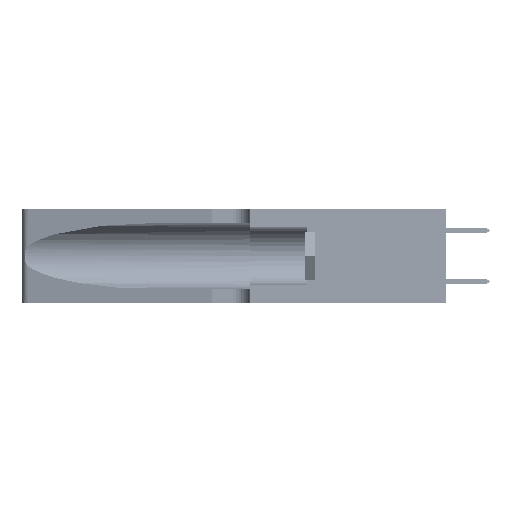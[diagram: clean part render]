
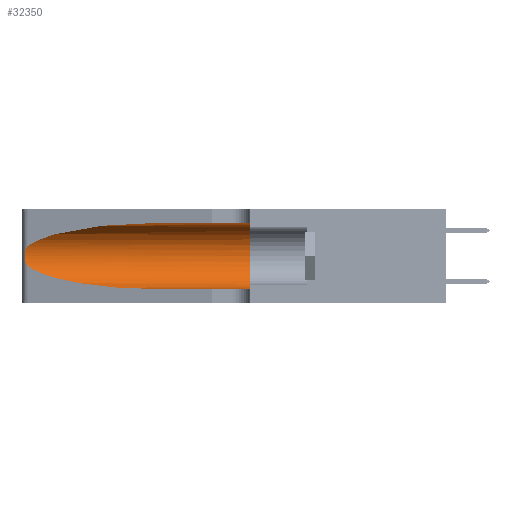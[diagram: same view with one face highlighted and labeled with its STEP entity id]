
A CAD part, left-side view. The second image highlights one B-rep face of the part: STEP entity #32350.
In plain terms, the highlighted cylindrical face has radius 3.308 mm (diameter 6.617 mm), a partial arc.
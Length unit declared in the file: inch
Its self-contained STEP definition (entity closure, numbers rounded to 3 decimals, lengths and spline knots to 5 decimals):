
#1364 = VERTEX_POINT ( 'NONE', #30475 ) ;
#2214 = CARTESIAN_POINT ( 'NONE',  ( 0.26075, 1.23896, 0.19203 ) ) ;
#2398 = CARTESIAN_POINT ( 'NONE',  ( 0.26017, 1.23833, 0.17102 ) ) ;
#4324 = FACE_OUTER_BOUND ( 'NONE', #38369, .T. ) ;
#5313 = CARTESIAN_POINT ( 'NONE',  ( 0.25487, 1.22718, 0.14631 ) ) ;
#6065 = EDGE_CURVE ( 'NONE', #1364, #43040, #25121, .T. ) ;
#6328 = CARTESIAN_POINT ( 'NONE',  ( 0.26075, 1.23896, 0.178 ) ) ;
#8182 = ORIENTED_EDGE ( 'NONE', *, *, #6065, .T. ) ;
#8504 = LINE ( 'NONE', #25974, #45544 ) ;
#8537 = AXIS2_PLACEMENT_3D ( 'NONE', #38284, #22401, #14534 ) ;
#9235 = CARTESIAN_POINT ( 'NONE',  ( 0.2373, 1.15595, 0.08982 ) ) ;
#9732 = CARTESIAN_POINT ( 'NONE',  ( 0.25639, 1.23186, 0.15144 ) ) ;
#9912 = CARTESIAN_POINT ( 'NONE',  ( 0.25789, 1.23486, 0.15765 ) ) ;
#14534 = DIRECTION ( 'NONE',  ( 0., 0., 1. ) ) ;
#15057 = ORIENTED_EDGE ( 'NONE', *, *, #47075, .T. ) ;
#15296 = CARTESIAN_POINT ( 'NONE',  ( 0.2373, 1.15595, 0.28018 ) ) ;
#15725 = CIRCLE ( 'NONE', #8537, 0.13025 ) ;
#16176 = CARTESIAN_POINT ( 'NONE',  ( 0.1305, 0.35, 0.05475 ) ) ;
#16829 = VERTEX_POINT ( 'NONE', #16176 ) ;
#17794 = DIRECTION ( 'NONE',  ( 0., -1., 0. ) ) ;
#18104 = CARTESIAN_POINT ( 'NONE',  ( 0.25555, 1.22994, 0.2215 ) ) ;
#18462 = CARTESIAN_POINT ( 'NONE',  ( 0.25487, 1.22718, 0.22369 ) ) ;
#18672 = EDGE_CURVE ( 'NONE', #46825, #24835, #45081, .T. ) ;
#20918 = CYLINDRICAL_SURFACE ( 'NONE', #23508, 0.13025 ) ;
#21162 = CARTESIAN_POINT ( 'NONE',  ( 0.1305, 1.61858, 0.05475 ) ) ;
#21567 = CARTESIAN_POINT ( 'NONE',  ( 0.18966, 0.96281, 0.05475 ) ) ;
#22038 = DIRECTION ( 'NONE',  ( 0., -1., 0. ) ) ;
#22401 = DIRECTION ( 'NONE',  ( 0., 1., 0. ) ) ;
#22582 = CARTESIAN_POINT ( 'NONE',  ( 0.25856, 1.23593, 0.16098 ) ) ;
#23114 = ORIENTED_EDGE ( 'NONE', *, *, #18672, .T. ) ;
#23508 = AXIS2_PLACEMENT_3D ( 'NONE', #42063, #17794, #31004 ) ;
#24835 = VERTEX_POINT ( 'NONE', #51493 ) ;
#24885 = ORIENTED_EDGE ( 'NONE', *, *, #35808, .F. ) ;
#25121 =( BOUNDED_CURVE ( )  B_SPLINE_CURVE ( 3, ( #5313, #9235, #21567, #42420 ),
 .UNSPECIFIED., .F., .F. ) 
 B_SPLINE_CURVE_WITH_KNOTS ( ( 4, 4 ),
 ( 3.44316, 4.71239 ),
 .UNSPECIFIED. ) 
 CURVE ( )  GEOMETRIC_REPRESENTATION_ITEM ( )  RATIONAL_B_SPLINE_CURVE ( ( 1., 0.87, 0.87, 1. ) ) 
 REPRESENTATION_ITEM ( '' )  );
#25974 = CARTESIAN_POINT ( 'NONE',  ( 0.1305, 1.61858, 0.31525 ) ) ;
#26861 = CARTESIAN_POINT ( 'NONE',  ( 0.25854, 1.2359, 0.20912 ) ) ;
#26919 = CARTESIAN_POINT ( 'NONE',  ( 0.18966, 0.96281, 0.31525 ) ) ;
#27288 = CARTESIAN_POINT ( 'NONE',  ( 0.1305, 0.72297, 0.31525 ) ) ;
#28362 = CARTESIAN_POINT ( 'NONE',  ( 0.1305, 0.72297, 0.05475 ) ) ;
#28686 = CARTESIAN_POINT ( 'NONE',  ( 0.1305, 0.72297, 0.31525 ) ) ;
#29132 = VERTEX_POINT ( 'NONE', #37899 ) ;
#30475 = CARTESIAN_POINT ( 'NONE',  ( 0.25487, 1.22718, 0.14631 ) ) ;
#30959 = CARTESIAN_POINT ( 'NONE',  ( 0.25555, 1.22993, 0.14849 ) ) ;
#31004 = DIRECTION ( 'NONE',  ( 0., 0., -1. ) ) ;
#32350 = ADVANCED_FACE ( 'NONE', ( #4324 ), #20918, .F. ) ;
#35808 = EDGE_CURVE ( 'NONE', #29132, #16829, #15725, .T. ) ;
#35902 = EDGE_CURVE ( 'NONE', #24835, #1364, #49912, .T. ) ;
#37899 = CARTESIAN_POINT ( 'NONE',  ( 0.1305, 0.35, 0.31525 ) ) ;
#37924 = EDGE_CURVE ( 'NONE', #46825, #29132, #8504, .T. ) ;
#38284 = CARTESIAN_POINT ( 'NONE',  ( 0.1305, 0.35, 0.185 ) ) ;
#38369 = EDGE_LOOP ( 'NONE', ( #23114, #41215, #8182, #15057, #24885, #42356 ) ) ;
#38619 = CARTESIAN_POINT ( 'NONE',  ( 0.26018, 1.23835, 0.19895 ) ) ;
#39205 = CARTESIAN_POINT ( 'NONE',  ( 0.25487, 1.22718, 0.22369 ) ) ;
#39246 = VECTOR ( 'NONE', #49731, 39.37008 ) ;
#41215 = ORIENTED_EDGE ( 'NONE', *, *, #35902, .T. ) ;
#42063 = CARTESIAN_POINT ( 'NONE',  ( 0.1305, 1.61858, 0.185 ) ) ;
#42356 = ORIENTED_EDGE ( 'NONE', *, *, #37924, .F. ) ;
#42420 = CARTESIAN_POINT ( 'NONE',  ( 0.1305, 0.72297, 0.05475 ) ) ;
#43040 = VERTEX_POINT ( 'NONE', #28362 ) ;
#45081 =( BOUNDED_CURVE ( )  B_SPLINE_CURVE ( 3, ( #27288, #26919, #15296, #39205 ),
 .UNSPECIFIED., .F., .F. ) 
 B_SPLINE_CURVE_WITH_KNOTS ( ( 4, 4 ),
 ( 1.5708, 2.84003 ),
 .UNSPECIFIED. ) 
 CURVE ( )  GEOMETRIC_REPRESENTATION_ITEM ( )  RATIONAL_B_SPLINE_CURVE ( ( 1., 0.87, 0.87, 1. ) ) 
 REPRESENTATION_ITEM ( '' )  );
#45544 = VECTOR ( 'NONE', #22038, 39.37008 ) ;
#46670 = CARTESIAN_POINT ( 'NONE',  ( 0.25487, 1.22718, 0.14631 ) ) ;
#46825 = VERTEX_POINT ( 'NONE', #28686 ) ;
#47029 = CARTESIAN_POINT ( 'NONE',  ( 0.25787, 1.23484, 0.2124 ) ) ;
#47075 = EDGE_CURVE ( 'NONE', #43040, #16829, #48251, .T. ) ;
#48251 = LINE ( 'NONE', #21162, #39246 ) ;
#49731 = DIRECTION ( 'NONE',  ( 0., -1., 0. ) ) ;
#49912 = B_SPLINE_CURVE_WITH_KNOTS ( 'NONE', 3,
 ( #18462, #18104, #50811, #47029, #26861, #38619, #2214, #6328, #2398, #22582, #9912, #9732, #30959, #46670 ),
 .UNSPECIFIED., .F., .F.,
 ( 4, 2, 2, 2, 2, 2, 4 ),
 ( 0., 0.00027, 0.00053, 0.00107, 0.0016, 0.00187, 0.00214 ),
 .UNSPECIFIED. ) ;
#50811 = CARTESIAN_POINT ( 'NONE',  ( 0.25639, 1.23184, 0.21858 ) ) ;
#51493 = CARTESIAN_POINT ( 'NONE',  ( 0.25487, 1.22718, 0.22369 ) ) ;
